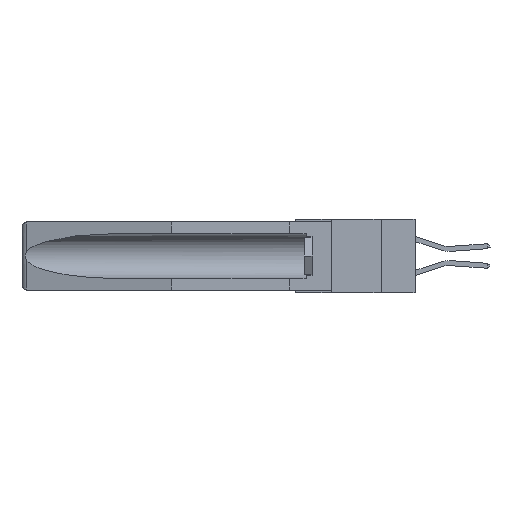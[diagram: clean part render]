
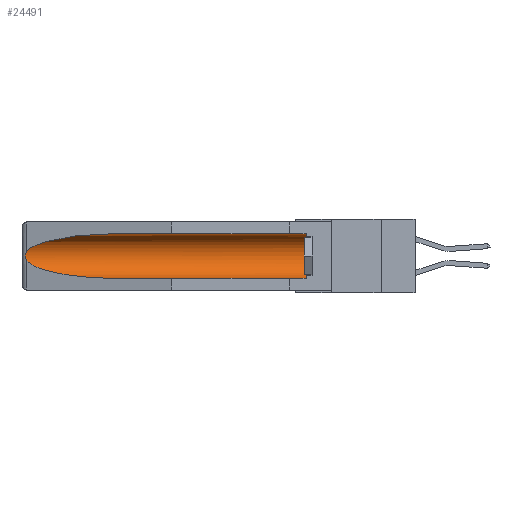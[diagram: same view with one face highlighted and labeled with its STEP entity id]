
A CAD part, left-side view. The second image highlights one B-rep face of the part: STEP entity #24491.
In plain terms, the highlighted cylindrical face has radius 2.857 mm (diameter 5.715 mm), a partial arc.
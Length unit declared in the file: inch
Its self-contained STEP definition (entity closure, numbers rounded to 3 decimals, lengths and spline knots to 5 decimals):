
#169 = CARTESIAN_POINT ( 'NONE',  ( 0.26654, 1.53092, -0.15636 ) ) ;
#1530 = CARTESIAN_POINT ( 'NONE',  ( 0.26537, 1.52718, -0.19328 ) ) ;
#1931 = AXIS2_PLACEMENT_3D ( 'NONE', #22567, #22469, #24760 ) ;
#2353 = ORIENTED_EDGE ( 'NONE', *, *, #29269, .T. ) ;
#2724 = AXIS2_PLACEMENT_3D ( 'NONE', #4597, #8011, #16610 ) ;
#2928 = VECTOR ( 'NONE', #11164, 39.37008 ) ;
#3002 = CARTESIAN_POINT ( 'NONE',  ( 0.26537, 1.52718, -0.14972 ) ) ;
#3242 = CARTESIAN_POINT ( 'NONE',  ( 0.25451, 1.48313, -0.09465 ) ) ;
#4104 = EDGE_CURVE ( 'NONE', #29022, #24009, #4671, .T. ) ;
#4551 = DIRECTION ( 'NONE',  ( 0., 1., 0. ) ) ;
#4597 = CARTESIAN_POINT ( 'NONE',  ( 0.155, -0.30754, -0.1715 ) ) ;
#4637 = CARTESIAN_POINT ( 'NONE',  ( 0.2673, 1.53269, -0.17917 ) ) ;
#4671 = LINE ( 'NONE', #29333, #2928 ) ;
#6109 = EDGE_CURVE ( 'NONE', #10095, #28975, #14544, .T. ) ;
#6631 = B_SPLINE_CURVE_WITH_KNOTS ( 'NONE', 3,
 ( #18049, #27476, #169, #20265, #9028, #20457, #4637, #24905, #11321, #27190 ),
 .UNSPECIFIED., .F., .F.,
 ( 4, 2, 2, 2, 4 ),
 ( 0., 0.00029, 0.00058, 0.00087, 0.00117 ),
 .UNSPECIFIED. ) ;
#7282 = CIRCLE ( 'NONE', #1931, 0.1125 ) ;
#8011 = DIRECTION ( 'NONE',  ( 0., 1., 0. ) ) ;
#8397 = CARTESIAN_POINT ( 'NONE',  ( 0.155, 0.126, -0.059 ) ) ;
#9028 = CARTESIAN_POINT ( 'NONE',  ( 0.2675, 1.53308, -0.16763 ) ) ;
#9341 = EDGE_CURVE ( 'NONE', #29022, #10095, #7282, .T. ) ;
#9693 = VERTEX_POINT ( 'NONE', #3002 ) ;
#10095 = VERTEX_POINT ( 'NONE', #8397 ) ;
#11164 = DIRECTION ( 'NONE',  ( 0., 1., 0. ) ) ;
#11321 = CARTESIAN_POINT ( 'NONE',  ( 0.26597, 1.5296, -0.19026 ) ) ;
#13284 = EDGE_LOOP ( 'NONE', ( #27323, #27806, #2353, #15831, #24493, #26523 ) ) ;
#13596 = CARTESIAN_POINT ( 'NONE',  ( 0.21114, 1.30732, -0.284 ) ) ;
#13692 = CARTESIAN_POINT ( 'NONE',  ( 0.155, 1.07973, -0.284 ) ) ;
#13777 = CARTESIAN_POINT ( 'NONE',  ( 0.26537, 1.52718, -0.19328 ) ) ;
#14544 = LINE ( 'NONE', #20670, #16308 ) ;
#15355 =( BOUNDED_CURVE ( )  B_SPLINE_CURVE ( 3, ( #13777, #25210, #13596, #13692 ),
 .UNSPECIFIED., .F., .F. ) 
 B_SPLINE_CURVE_WITH_KNOTS ( ( 4, 4 ),
 ( 0.1948, 1.5708 ),
 .UNSPECIFIED. ) 
 CURVE ( )  GEOMETRIC_REPRESENTATION_ITEM ( )  RATIONAL_B_SPLINE_CURVE ( ( 1., 0.848, 0.848, 1. ) ) 
 REPRESENTATION_ITEM ( '' )  );
#15831 = ORIENTED_EDGE ( 'NONE', *, *, #4104, .F. ) ;
#16308 = VECTOR ( 'NONE', #4551, 39.37008 ) ;
#16610 = DIRECTION ( 'NONE',  ( 0., 0., 1. ) ) ;
#17506 = FACE_OUTER_BOUND ( 'NONE', #13284, .T. ) ;
#18049 = CARTESIAN_POINT ( 'NONE',  ( 0.26537, 1.52718, -0.14972 ) ) ;
#19131 = CARTESIAN_POINT ( 'NONE',  ( 0.26537, 1.52718, -0.14972 ) ) ;
#20265 = CARTESIAN_POINT ( 'NONE',  ( 0.2673, 1.5327, -0.16383 ) ) ;
#20364 = EDGE_CURVE ( 'NONE', #9693, #23726, #6631, .T. ) ;
#20457 = CARTESIAN_POINT ( 'NONE',  ( 0.2675, 1.53308, -0.17534 ) ) ;
#20670 = CARTESIAN_POINT ( 'NONE',  ( 0.155, -0.30754, -0.059 ) ) ;
#21803 = CYLINDRICAL_SURFACE ( 'NONE', #2724, 0.1125 ) ;
#22165 = CARTESIAN_POINT ( 'NONE',  ( 0.155, 1.07973, -0.059 ) ) ;
#22469 = DIRECTION ( 'NONE',  ( 0., -1., 0. ) ) ;
#22471 =( BOUNDED_CURVE ( )  B_SPLINE_CURVE ( 3, ( #22872, #23597, #3242, #19131 ),
 .UNSPECIFIED., .F., .T. ) 
 B_SPLINE_CURVE_WITH_KNOTS ( ( 4, 4 ),
 ( 4.71239, 6.08839 ),
 .UNSPECIFIED. ) 
 CURVE ( )  GEOMETRIC_REPRESENTATION_ITEM ( )  RATIONAL_B_SPLINE_CURVE ( ( 1., 0.848, 0.848, 1. ) ) 
 REPRESENTATION_ITEM ( '' )  );
#22567 = CARTESIAN_POINT ( 'NONE',  ( 0.155, 0.126, -0.1715 ) ) ;
#22872 = CARTESIAN_POINT ( 'NONE',  ( 0.155, 1.07973, -0.059 ) ) ;
#23597 = CARTESIAN_POINT ( 'NONE',  ( 0.21114, 1.30732, -0.059 ) ) ;
#23726 = VERTEX_POINT ( 'NONE', #1530 ) ;
#24009 = VERTEX_POINT ( 'NONE', #28197 ) ;
#24491 = ADVANCED_FACE ( 'NONE', ( #17506 ), #21803, .F. ) ;
#24493 = ORIENTED_EDGE ( 'NONE', *, *, #9341, .T. ) ;
#24760 = DIRECTION ( 'NONE',  ( 0., 0., 1. ) ) ;
#24905 = CARTESIAN_POINT ( 'NONE',  ( 0.26655, 1.53094, -0.18657 ) ) ;
#24993 = EDGE_CURVE ( 'NONE', #28975, #9693, #22471, .T. ) ;
#25012 = CARTESIAN_POINT ( 'NONE',  ( 0.155, 0.126, -0.284 ) ) ;
#25210 = CARTESIAN_POINT ( 'NONE',  ( 0.25451, 1.48313, -0.24835 ) ) ;
#26523 = ORIENTED_EDGE ( 'NONE', *, *, #6109, .T. ) ;
#27190 = CARTESIAN_POINT ( 'NONE',  ( 0.26537, 1.52718, -0.19328 ) ) ;
#27323 = ORIENTED_EDGE ( 'NONE', *, *, #24993, .T. ) ;
#27476 = CARTESIAN_POINT ( 'NONE',  ( 0.26597, 1.52961, -0.15275 ) ) ;
#27806 = ORIENTED_EDGE ( 'NONE', *, *, #20364, .T. ) ;
#28197 = CARTESIAN_POINT ( 'NONE',  ( 0.155, 1.07973, -0.284 ) ) ;
#28975 = VERTEX_POINT ( 'NONE', #22165 ) ;
#29022 = VERTEX_POINT ( 'NONE', #25012 ) ;
#29269 = EDGE_CURVE ( 'NONE', #23726, #24009, #15355, .T. ) ;
#29333 = CARTESIAN_POINT ( 'NONE',  ( 0.155, -0.30754, -0.284 ) ) ;
